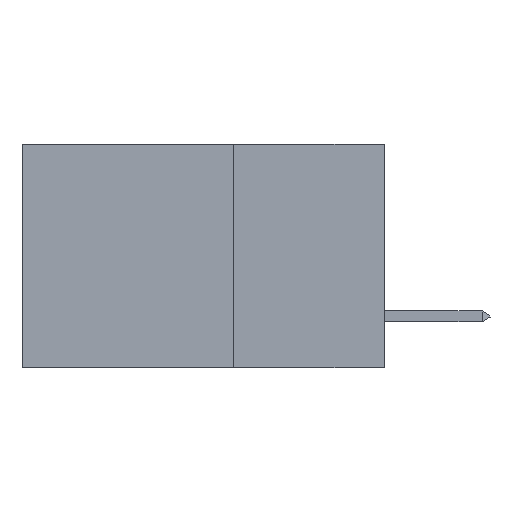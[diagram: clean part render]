
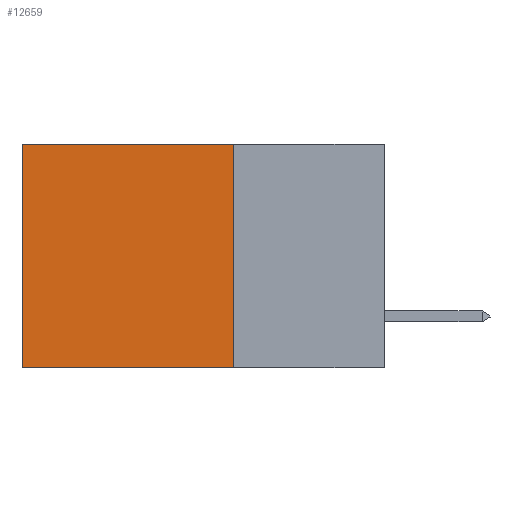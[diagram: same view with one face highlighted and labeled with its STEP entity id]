
A CAD part, left-side view. The second image highlights one B-rep face of the part: STEP entity #12659.
In plain terms, the highlighted planar face has unit normal (-1, 0, 0).
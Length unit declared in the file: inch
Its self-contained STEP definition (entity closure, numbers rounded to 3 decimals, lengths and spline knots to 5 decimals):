
#2610 = FACE_OUTER_BOUND ( 'NONE', #11612, .T. ) ;
#2762 = VERTEX_POINT ( 'NONE', #9911 ) ;
#3712 = DIRECTION ( 'NONE',  ( 0., 0., -1. ) ) ;
#3848 = VECTOR ( 'NONE', #32726, 39.37008 ) ;
#3878 = ORIENTED_EDGE ( 'NONE', *, *, #39477, .T. ) ;
#4073 = CARTESIAN_POINT ( 'NONE',  ( 0.2875, 0.25, 0. ) ) ;
#4131 = CARTESIAN_POINT ( 'NONE',  ( 0.2875, 0.25, 0. ) ) ;
#4495 = VERTEX_POINT ( 'NONE', #30823 ) ;
#4819 = CARTESIAN_POINT ( 'NONE',  ( 0.2875, 0.25, 0. ) ) ;
#5101 = ORIENTED_EDGE ( 'NONE', *, *, #8315, .F. ) ;
#7527 = CARTESIAN_POINT ( 'NONE',  ( 0.2875, 0.6, 0. ) ) ;
#7760 = ORIENTED_EDGE ( 'NONE', *, *, #21446, .F. ) ;
#8207 = DIRECTION ( 'NONE',  ( 0., 0., -1. ) ) ;
#8209 = CARTESIAN_POINT ( 'NONE',  ( 0.2875, 0.25, -0.37 ) ) ;
#8315 = EDGE_CURVE ( 'NONE', #4495, #2762, #23521, .T. ) ;
#9911 = CARTESIAN_POINT ( 'NONE',  ( 0.2875, 0.6, -0.37 ) ) ;
#11612 = EDGE_LOOP ( 'NONE', ( #3878, #5101, #7760, #39881 ) ) ;
#12659 = ADVANCED_FACE ( 'NONE', ( #2610 ), #30974, .F. ) ;
#14674 = LINE ( 'NONE', #7527, #33946 ) ;
#15895 = LINE ( 'NONE', #4131, #20592 ) ;
#20592 = VECTOR ( 'NONE', #3712, 39.37008 ) ;
#21125 = DIRECTION ( 'NONE',  ( 0., 1., 0. ) ) ;
#21446 = EDGE_CURVE ( 'NONE', #32280, #4495, #15895, .T. ) ;
#23521 = LINE ( 'NONE', #8209, #3848 ) ;
#24016 = CARTESIAN_POINT ( 'NONE',  ( 0.2875, 0.25, 0. ) ) ;
#24518 = AXIS2_PLACEMENT_3D ( 'NONE', #4819, #28621, #8207 ) ;
#26171 = LINE ( 'NONE', #4073, #34179 ) ;
#28621 = DIRECTION ( 'NONE',  ( 1., 0., 0. ) ) ;
#29207 = VERTEX_POINT ( 'NONE', #30317 ) ;
#30317 = CARTESIAN_POINT ( 'NONE',  ( 0.2875, 0.6, 0. ) ) ;
#30823 = CARTESIAN_POINT ( 'NONE',  ( 0.2875, 0.25, -0.37 ) ) ;
#30974 = PLANE ( 'NONE',  #24518 ) ;
#32280 = VERTEX_POINT ( 'NONE', #24016 ) ;
#32726 = DIRECTION ( 'NONE',  ( 0., 1., 0. ) ) ;
#33946 = VECTOR ( 'NONE', #35273, 39.37008 ) ;
#34179 = VECTOR ( 'NONE', #21125, 39.37008 ) ;
#35273 = DIRECTION ( 'NONE',  ( 0., 0., -1. ) ) ;
#36524 = EDGE_CURVE ( 'NONE', #32280, #29207, #26171, .T. ) ;
#39477 = EDGE_CURVE ( 'NONE', #29207, #2762, #14674, .T. ) ;
#39881 = ORIENTED_EDGE ( 'NONE', *, *, #36524, .T. ) ;
